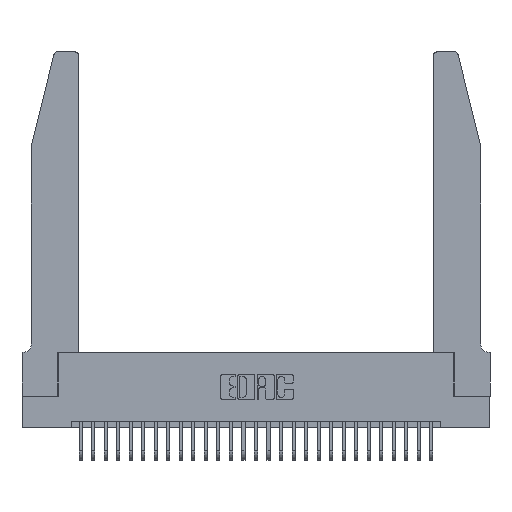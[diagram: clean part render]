
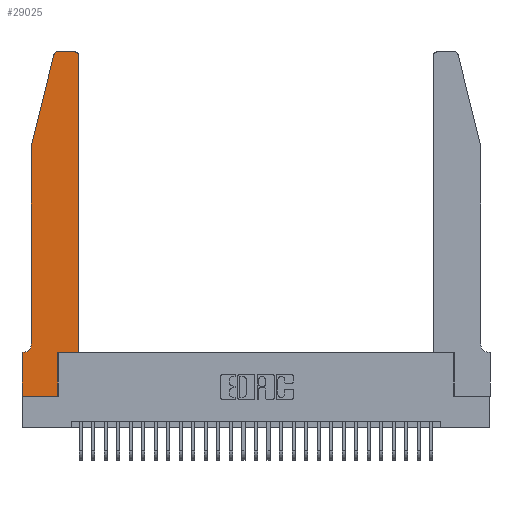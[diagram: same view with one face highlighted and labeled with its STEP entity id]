
A CAD part, top view. The second image highlights one B-rep face of the part: STEP entity #29025.
In plain terms, the highlighted planar face has unit normal (0, 0, 1).
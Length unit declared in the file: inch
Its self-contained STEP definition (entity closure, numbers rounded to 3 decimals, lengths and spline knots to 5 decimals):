
#281 = CARTESIAN_POINT ( 'NONE',  ( 0.2865, 0., 0.37 ) ) ;
#572 = ORIENTED_EDGE ( 'NONE', *, *, #15084, .T. ) ;
#831 = AXIS2_PLACEMENT_3D ( 'NONE', #11875, #9584, #23871 ) ;
#945 = ORIENTED_EDGE ( 'NONE', *, *, #14588, .T. ) ;
#1669 = DIRECTION ( 'NONE',  ( 1., 0., 0. ) ) ;
#3055 = DIRECTION ( 'NONE',  ( 0., -1., 0. ) ) ;
#3271 = CARTESIAN_POINT ( 'NONE',  ( 0.2865, 0.35, 0.37 ) ) ;
#3349 = VERTEX_POINT ( 'NONE', #18865 ) ;
#3912 = CARTESIAN_POINT ( 'NONE',  ( 0.0055, 0.42, 0.37 ) ) ;
#3986 = LINE ( 'NONE', #15574, #4760 ) ;
#3992 = CARTESIAN_POINT ( 'NONE',  ( 0., 0., 0.37 ) ) ;
#4642 = VECTOR ( 'NONE', #10648, 39.37008 ) ;
#4760 = VECTOR ( 'NONE', #21299, 39.37008 ) ;
#4963 = LINE ( 'NONE', #13046, #11371 ) ;
#5166 = CARTESIAN_POINT ( 'NONE',  ( 0.4505, 0.35, 0.37 ) ) ;
#5388 = CARTESIAN_POINT ( 'NONE',  ( 0.4205, 2.75, 0.37 ) ) ;
#5400 = DIRECTION ( 'NONE',  ( 0., 1., 0. ) ) ;
#6099 = CIRCLE ( 'NONE', #831, 0.03 ) ;
#6564 = AXIS2_PLACEMENT_3D ( 'NONE', #3912, #23078, #15952 ) ;
#6779 = CARTESIAN_POINT ( 'NONE',  ( 0., 0.35, 0.37 ) ) ;
#7696 = DIRECTION ( 'NONE',  ( 0., 1., 0. ) ) ;
#7886 = CARTESIAN_POINT ( 'NONE',  ( 0.0755, 0.42, 0.37 ) ) ;
#7900 = EDGE_CURVE ( 'NONE', #24370, #16903, #10906, .T. ) ;
#7944 = CARTESIAN_POINT ( 'NONE',  ( 0.4505, 2.72, 0.37 ) ) ;
#7953 = LINE ( 'NONE', #3992, #28487 ) ;
#8012 = EDGE_CURVE ( 'NONE', #8697, #14317, #28802, .T. ) ;
#8143 = CARTESIAN_POINT ( 'NONE',  ( 0.4505, 0.35, 0.37 ) ) ;
#8271 = VERTEX_POINT ( 'NONE', #7886 ) ;
#8697 = VERTEX_POINT ( 'NONE', #11413 ) ;
#8763 = DIRECTION ( 'NONE',  ( 1., 0., 0. ) ) ;
#8950 = DIRECTION ( 'NONE',  ( 1., 0., 0. ) ) ;
#9223 = VERTEX_POINT ( 'NONE', #28940 ) ;
#9409 = ORIENTED_EDGE ( 'NONE', *, *, #24014, .T. ) ;
#9584 = DIRECTION ( 'NONE',  ( 0., 0., 1. ) ) ;
#9745 = ORIENTED_EDGE ( 'NONE', *, *, #7900, .T. ) ;
#10326 = CARTESIAN_POINT ( 'NONE',  ( 0., 0., 0.37 ) ) ;
#10644 = DIRECTION ( 'NONE',  ( -1., 0., 0. ) ) ;
#10648 = DIRECTION ( 'NONE',  ( 1., 0., 0. ) ) ;
#10906 = LINE ( 'NONE', #12094, #26971 ) ;
#11371 = VECTOR ( 'NONE', #10644, 39.37008 ) ;
#11413 = CARTESIAN_POINT ( 'NONE',  ( 0.4505, 0.35, 0.37 ) ) ;
#11455 = ORIENTED_EDGE ( 'NONE', *, *, #27561, .T. ) ;
#11462 = CARTESIAN_POINT ( 'NONE',  ( 0.25487, 2.72718, 0.37 ) ) ;
#11875 = CARTESIAN_POINT ( 'NONE',  ( 0.284, 2.72, 0.37 ) ) ;
#11991 = VERTEX_POINT ( 'NONE', #6779 ) ;
#12094 = CARTESIAN_POINT ( 'NONE',  ( 0.0755, 2., 0.37 ) ) ;
#12417 = CIRCLE ( 'NONE', #6564, 0.07 ) ;
#12548 = VECTOR ( 'NONE', #29602, 39.37008 ) ;
#12934 = EDGE_CURVE ( 'NONE', #16903, #8271, #3986, .T. ) ;
#13046 = CARTESIAN_POINT ( 'NONE',  ( 0.2605, 2.75, 0.37 ) ) ;
#13134 = ORIENTED_EDGE ( 'NONE', *, *, #19286, .T. ) ;
#13256 = CIRCLE ( 'NONE', #20512, 0.03 ) ;
#13272 = VECTOR ( 'NONE', #3055, 39.37008 ) ;
#14134 = VERTEX_POINT ( 'NONE', #10326 ) ;
#14317 = VERTEX_POINT ( 'NONE', #7944 ) ;
#14588 = EDGE_CURVE ( 'NONE', #14970, #8697, #26031, .T. ) ;
#14970 = VERTEX_POINT ( 'NONE', #27825 ) ;
#15084 = EDGE_CURVE ( 'NONE', #14317, #28302, #13256, .T. ) ;
#15574 = CARTESIAN_POINT ( 'NONE',  ( 0.0755, 2., 0.37 ) ) ;
#15699 = AXIS2_PLACEMENT_3D ( 'NONE', #16095, #28326, #1669 ) ;
#15952 = DIRECTION ( 'NONE',  ( -1., 0., 0. ) ) ;
#16095 = CARTESIAN_POINT ( 'NONE',  ( 0., 0.35, 0.37 ) ) ;
#16119 = EDGE_CURVE ( 'NONE', #14134, #17484, #7953, .T. ) ;
#16206 = DIRECTION ( 'NONE',  ( 0., 0., 1. ) ) ;
#16391 = EDGE_CURVE ( 'NONE', #8271, #9223, #12417, .T. ) ;
#16569 = ORIENTED_EDGE ( 'NONE', *, *, #12934, .T. ) ;
#16903 = VERTEX_POINT ( 'NONE', #23972 ) ;
#17484 = VERTEX_POINT ( 'NONE', #281 ) ;
#17693 = ORIENTED_EDGE ( 'NONE', *, *, #8012, .T. ) ;
#18865 = CARTESIAN_POINT ( 'NONE',  ( 0.284, 2.75, 0.37 ) ) ;
#19199 = EDGE_LOOP ( 'NONE', ( #25008, #25811, #9745, #16569, #24253, #11455, #9409, #30104, #13134, #945, #17693, #572 ) ) ;
#19286 = EDGE_CURVE ( 'NONE', #17484, #14970, #29836, .T. ) ;
#20512 = AXIS2_PLACEMENT_3D ( 'NONE', #21109, #16206, #8950 ) ;
#20545 = VECTOR ( 'NONE', #7696, 39.37008 ) ;
#20790 = PLANE ( 'NONE',  #15699 ) ;
#21109 = CARTESIAN_POINT ( 'NONE',  ( 0.4205, 2.72, 0.37 ) ) ;
#21299 = DIRECTION ( 'NONE',  ( 0., -1., 0. ) ) ;
#22970 = LINE ( 'NONE', #27321, #12548 ) ;
#23078 = DIRECTION ( 'NONE',  ( 0., 0., -1. ) ) ;
#23486 = VECTOR ( 'NONE', #5400, 39.37008 ) ;
#23871 = DIRECTION ( 'NONE',  ( 1., 0., 0. ) ) ;
#23972 = CARTESIAN_POINT ( 'NONE',  ( 0.0755, 2., 0.37 ) ) ;
#24014 = EDGE_CURVE ( 'NONE', #11991, #14134, #29321, .T. ) ;
#24253 = ORIENTED_EDGE ( 'NONE', *, *, #16391, .T. ) ;
#24370 = VERTEX_POINT ( 'NONE', #11462 ) ;
#25008 = ORIENTED_EDGE ( 'NONE', *, *, #25227, .T. ) ;
#25227 = EDGE_CURVE ( 'NONE', #28302, #3349, #4963, .T. ) ;
#25436 = EDGE_CURVE ( 'NONE', #3349, #24370, #6099, .T. ) ;
#25811 = ORIENTED_EDGE ( 'NONE', *, *, #25436, .T. ) ;
#25913 = FACE_OUTER_BOUND ( 'NONE', #19199, .T. ) ;
#26031 = LINE ( 'NONE', #8143, #4642 ) ;
#26304 = DIRECTION ( 'NONE',  ( -0.239, -0.971, 0. ) ) ;
#26971 = VECTOR ( 'NONE', #26304, 39.37008 ) ;
#27045 = CARTESIAN_POINT ( 'NONE',  ( 0., 0., 0.37 ) ) ;
#27321 = CARTESIAN_POINT ( 'NONE',  ( 0.0755, 0.35, 0.37 ) ) ;
#27561 = EDGE_CURVE ( 'NONE', #9223, #11991, #22970, .T. ) ;
#27825 = CARTESIAN_POINT ( 'NONE',  ( 0.2865, 0.35, 0.37 ) ) ;
#28302 = VERTEX_POINT ( 'NONE', #5388 ) ;
#28326 = DIRECTION ( 'NONE',  ( 0., 0., 1. ) ) ;
#28487 = VECTOR ( 'NONE', #8763, 39.37008 ) ;
#28802 = LINE ( 'NONE', #5166, #20545 ) ;
#28940 = CARTESIAN_POINT ( 'NONE',  ( 0.0055, 0.35, 0.37 ) ) ;
#29025 = ADVANCED_FACE ( 'NONE', ( #25913 ), #20790, .T. ) ;
#29321 = LINE ( 'NONE', #27045, #13272 ) ;
#29602 = DIRECTION ( 'NONE',  ( -1., 0., 0. ) ) ;
#29836 = LINE ( 'NONE', #3271, #23486 ) ;
#30104 = ORIENTED_EDGE ( 'NONE', *, *, #16119, .T. ) ;
